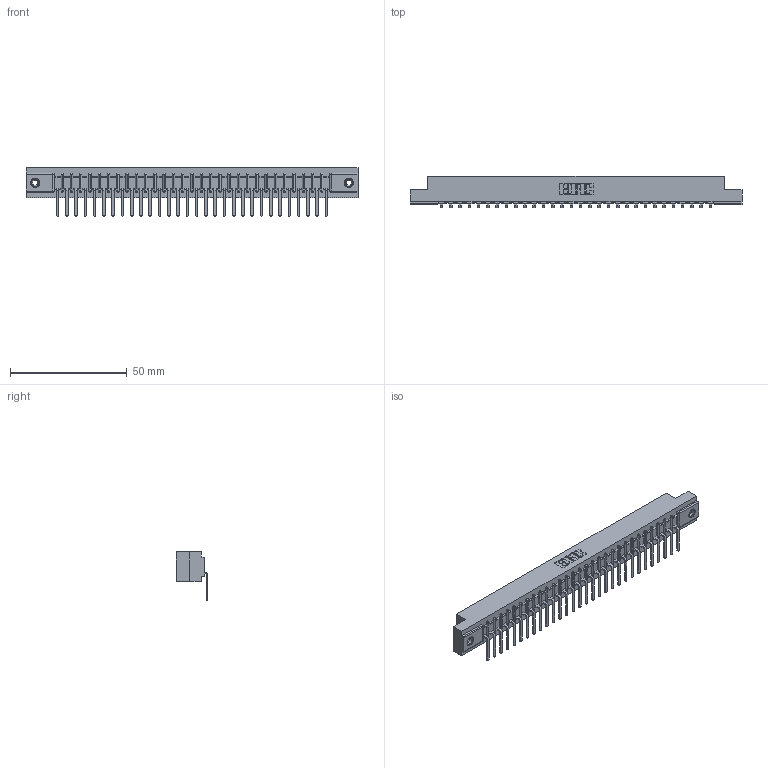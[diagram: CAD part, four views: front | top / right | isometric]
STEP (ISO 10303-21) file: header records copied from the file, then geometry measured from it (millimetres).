
FILE_DESCRIPTION (( 'STEP AP203' ), '1' );
FILE_NAME ('307-030-457-108.STEP', '2020-09-28T12:23:53', ( '' ), ( '' ), 'SwSTEP 2.0', 'SolidWorks 2020', '' );
FILE_SCHEMA (( 'CONFIG_CONTROL_DESIGN' ));
Length unit declared in the file: inch
Products named in the file (4): 345-250-001_345-250-003-102; 307 Part_.156 Dia Mounting Holes; 307-030-457-108; 307-290-002_557
Assembly tree (33 placements, depth 2):
  307-030-457-108
    307 Part_.156 Dia Mounting Holes
    307-290-002_557  x30
    345-250-001_345-250-003-102  x2
Bounding box: 141.88 x 13.32 x 20.66 mm (x, y, z)
Volume: 15168.4 mm3; surface area: 19355.3 mm2
Topology: 33 solids, 33 shells, 2549 faces, 7779 edges, 5094 vertices
Faces by surface type: plane 1512, cylinder 959, sphere 62, cone 12, torus 4
Entity records: 29237 total; most frequent: CARTESIAN_POINT 4911, ORIENTED_EDGE 4894, DIRECTION 4787, EDGE_CURVE 2447, LINE 1867, VECTOR 1867, VERTEX_POINT 1584, AXIS2_PLACEMENT_3D 1460
